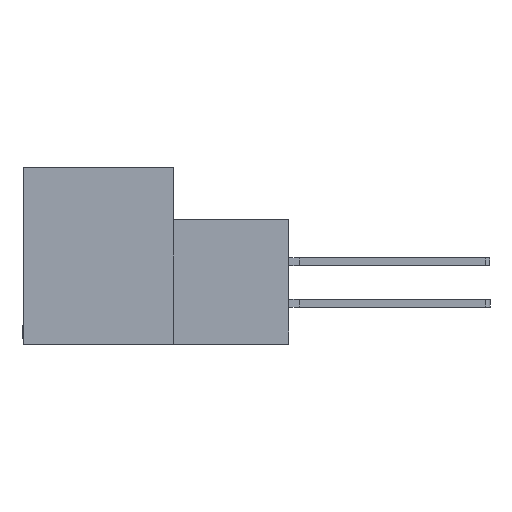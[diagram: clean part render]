
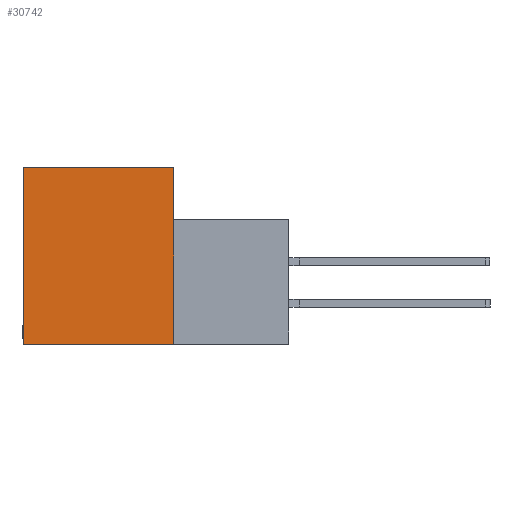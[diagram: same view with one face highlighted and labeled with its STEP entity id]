
A CAD part, left-side view. The second image highlights one B-rep face of the part: STEP entity #30742.
In plain terms, the highlighted planar face has unit normal (-1, 0, 0).
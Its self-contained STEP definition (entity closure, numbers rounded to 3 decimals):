
#604 = DIRECTION ( 'NONE',  ( 1., 0., 0. ) ) ;
#1524 = VERTEX_POINT ( 'NONE', #21537 ) ;
#2635 = VERTEX_POINT ( 'NONE', #30891 ) ;
#3398 = ORIENTED_EDGE ( 'NONE', *, *, #18111, .F. ) ;
#4716 = CARTESIAN_POINT ( 'NONE',  ( 0., 11.506, 0. ) ) ;
#4744 = VERTEX_POINT ( 'NONE', #4716 ) ;
#6108 = CARTESIAN_POINT ( 'NONE',  ( 0., 0., 0. ) ) ;
#6925 = CARTESIAN_POINT ( 'NONE',  ( 0., 0., -13.487 ) ) ;
#7604 = LINE ( 'NONE', #12633, #8001 ) ;
#8001 = VECTOR ( 'NONE', #20267, 1000. ) ;
#8255 = DIRECTION ( 'NONE',  ( 0., 0., 1. ) ) ;
#8633 = EDGE_CURVE ( 'NONE', #4744, #1524, #7604, .T. ) ;
#8642 = LINE ( 'NONE', #26476, #18720 ) ;
#10727 = VECTOR ( 'NONE', #23034, 1000. ) ;
#11625 = VECTOR ( 'NONE', #8255, 1000. ) ;
#11655 = EDGE_CURVE ( 'NONE', #1524, #13551, #8642, .T. ) ;
#11670 = PLANE ( 'NONE',  #22193 ) ;
#12633 = CARTESIAN_POINT ( 'NONE',  ( 0., 11.506, 0. ) ) ;
#13196 = CARTESIAN_POINT ( 'NONE',  ( 0., 11.506, -13.487 ) ) ;
#13551 = VERTEX_POINT ( 'NONE', #6925 ) ;
#18111 = EDGE_CURVE ( 'NONE', #13551, #2635, #27543, .T. ) ;
#18636 = ORIENTED_EDGE ( 'NONE', *, *, #20545, .F. ) ;
#18720 = VECTOR ( 'NONE', #24113, 1000. ) ;
#19574 = LINE ( 'NONE', #13196, #11625 ) ;
#20267 = DIRECTION ( 'NONE',  ( 0., -1., 0. ) ) ;
#20545 = EDGE_CURVE ( 'NONE', #2635, #4744, #19574, .T. ) ;
#21537 = CARTESIAN_POINT ( 'NONE',  ( 0., 0., 0. ) ) ;
#22193 = AXIS2_PLACEMENT_3D ( 'NONE', #6108, #604, #30077 ) ;
#23034 = DIRECTION ( 'NONE',  ( 0., 1., 0. ) ) ;
#23149 = CARTESIAN_POINT ( 'NONE',  ( 0., -8.814, -13.487 ) ) ;
#24113 = DIRECTION ( 'NONE',  ( 0., 0., -1. ) ) ;
#26200 = FACE_OUTER_BOUND ( 'NONE', #34436, .T. ) ;
#26476 = CARTESIAN_POINT ( 'NONE',  ( 0., 0., 0. ) ) ;
#27071 = ORIENTED_EDGE ( 'NONE', *, *, #11655, .F. ) ;
#27543 = LINE ( 'NONE', #23149, #10727 ) ;
#30077 = DIRECTION ( 'NONE',  ( 0., 0., -1. ) ) ;
#30480 = ORIENTED_EDGE ( 'NONE', *, *, #8633, .F. ) ;
#30742 = ADVANCED_FACE ( 'NONE', ( #26200 ), #11670, .F. ) ;
#30891 = CARTESIAN_POINT ( 'NONE',  ( 0., 11.506, -13.487 ) ) ;
#34436 = EDGE_LOOP ( 'NONE', ( #3398, #27071, #30480, #18636 ) ) ;
